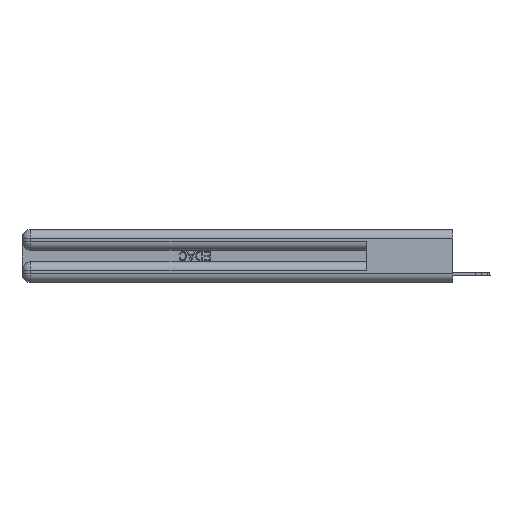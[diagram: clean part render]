
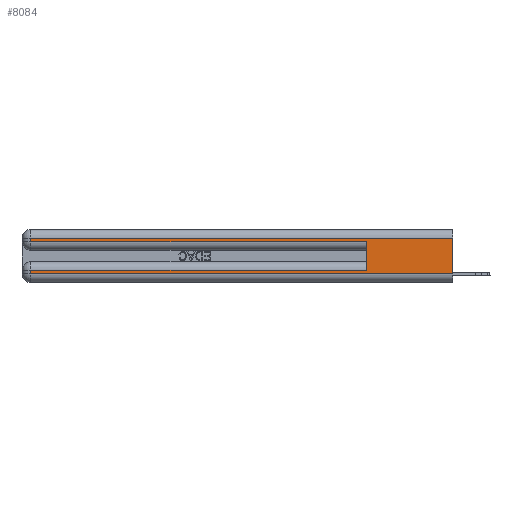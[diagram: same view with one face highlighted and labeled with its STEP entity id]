
A CAD part, left-side view. The second image highlights one B-rep face of the part: STEP entity #8084.
In plain terms, the highlighted planar face has unit normal (-1, 0, 0).
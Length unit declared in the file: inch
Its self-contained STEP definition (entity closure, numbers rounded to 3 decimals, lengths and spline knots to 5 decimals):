
#580 = CARTESIAN_POINT ( 'NONE',  ( 0., 2.94, 0.37 ) ) ;
#921 = CARTESIAN_POINT ( 'NONE',  ( 0., 0., 0.06 ) ) ;
#997 = CARTESIAN_POINT ( 'NONE',  ( 0., 0., 0.37 ) ) ;
#1278 = EDGE_CURVE ( 'NONE', #8071, #2235, #15853, .T. ) ;
#2235 = VERTEX_POINT ( 'NONE', #9827 ) ;
#2362 = CARTESIAN_POINT ( 'NONE',  ( 0., 0., 0.06 ) ) ;
#2391 = ORIENTED_EDGE ( 'NONE', *, *, #28402, .T. ) ;
#3231 = LINE ( 'NONE', #3820, #8167 ) ;
#3665 = DIRECTION ( 'NONE',  ( 0., 0., 1. ) ) ;
#3820 = CARTESIAN_POINT ( 'NONE',  ( 0., 0.6, 0.145 ) ) ;
#3840 = VECTOR ( 'NONE', #24887, 39.37008 ) ;
#4659 = ORIENTED_EDGE ( 'NONE', *, *, #1278, .T. ) ;
#4797 = ORIENTED_EDGE ( 'NONE', *, *, #5180, .T. ) ;
#5086 = VERTEX_POINT ( 'NONE', #6696 ) ;
#5180 = EDGE_CURVE ( 'NONE', #18033, #19035, #28185, .T. ) ;
#5186 = DIRECTION ( 'NONE',  ( 0., 0., -1. ) ) ;
#5324 = VECTOR ( 'NONE', #5186, 39.37008 ) ;
#5557 = CARTESIAN_POINT ( 'NONE',  ( 0., 0., 0.37 ) ) ;
#5672 = VERTEX_POINT ( 'NONE', #11124 ) ;
#5838 = CARTESIAN_POINT ( 'NONE',  ( 0., 2.94, 0.085 ) ) ;
#6696 = CARTESIAN_POINT ( 'NONE',  ( 0., 2.94, 0.06 ) ) ;
#7881 = EDGE_CURVE ( 'NONE', #8071, #9326, #16657, .T. ) ;
#7903 = CARTESIAN_POINT ( 'NONE',  ( 0., 0., 0.31 ) ) ;
#8071 = VERTEX_POINT ( 'NONE', #7903 ) ;
#8084 = ADVANCED_FACE ( 'NONE', ( #16611 ), #14813, .F. ) ;
#8167 = VECTOR ( 'NONE', #3665, 39.37008 ) ;
#9326 = VERTEX_POINT ( 'NONE', #2362 ) ;
#9507 = ORIENTED_EDGE ( 'NONE', *, *, #9837, .T. ) ;
#9827 = CARTESIAN_POINT ( 'NONE',  ( 0., 2.94, 0.31 ) ) ;
#9837 = EDGE_CURVE ( 'NONE', #5672, #10639, #11493, .T. ) ;
#9947 = EDGE_CURVE ( 'NONE', #18033, #10639, #3231, .T. ) ;
#9996 = DIRECTION ( 'NONE',  ( 0., 0., -1. ) ) ;
#10639 = VERTEX_POINT ( 'NONE', #11618 ) ;
#11124 = CARTESIAN_POINT ( 'NONE',  ( 0., 2.94, 0.285 ) ) ;
#11217 = EDGE_CURVE ( 'NONE', #5086, #9326, #11985, .T. ) ;
#11493 = LINE ( 'NONE', #27300, #27968 ) ;
#11618 = CARTESIAN_POINT ( 'NONE',  ( 0., 0.6, 0.285 ) ) ;
#11985 = LINE ( 'NONE', #921, #28981 ) ;
#12305 = DIRECTION ( 'NONE',  ( 0., 0., -1. ) ) ;
#12438 = LINE ( 'NONE', #12720, #20201 ) ;
#12720 = CARTESIAN_POINT ( 'NONE',  ( 0., 2.94, 0.37 ) ) ;
#12856 = AXIS2_PLACEMENT_3D ( 'NONE', #5557, #18840, #12305 ) ;
#13127 = ORIENTED_EDGE ( 'NONE', *, *, #23274, .T. ) ;
#13613 = CARTESIAN_POINT ( 'NONE',  ( 0., 0., 0.31 ) ) ;
#14120 = DIRECTION ( 'NONE',  ( 0., -1., 0. ) ) ;
#14813 = PLANE ( 'NONE',  #12856 ) ;
#15853 = LINE ( 'NONE', #13613, #3840 ) ;
#16119 = DIRECTION ( 'NONE',  ( 0., 1., 0. ) ) ;
#16597 = DIRECTION ( 'NONE',  ( 0., 0., -1. ) ) ;
#16611 = FACE_OUTER_BOUND ( 'NONE', #17131, .T. ) ;
#16657 = LINE ( 'NONE', #997, #23710 ) ;
#17131 = EDGE_LOOP ( 'NONE', ( #28133, #4659, #13127, #9507, #26102, #4797, #2391, #28627 ) ) ;
#18033 = VERTEX_POINT ( 'NONE', #26033 ) ;
#18586 = LINE ( 'NONE', #580, #5324 ) ;
#18673 = VECTOR ( 'NONE', #16119, 39.37008 ) ;
#18840 = DIRECTION ( 'NONE',  ( 1., 0., 0. ) ) ;
#19035 = VERTEX_POINT ( 'NONE', #5838 ) ;
#20201 = VECTOR ( 'NONE', #16597, 39.37008 ) ;
#21026 = DIRECTION ( 'NONE',  ( 0., -1., 0. ) ) ;
#23274 = EDGE_CURVE ( 'NONE', #2235, #5672, #12438, .T. ) ;
#23710 = VECTOR ( 'NONE', #9996, 39.37008 ) ;
#24887 = DIRECTION ( 'NONE',  ( 0., 1., 0. ) ) ;
#25144 = CARTESIAN_POINT ( 'NONE',  ( 0., 0., 0.085 ) ) ;
#26033 = CARTESIAN_POINT ( 'NONE',  ( 0., 0.6, 0.085 ) ) ;
#26102 = ORIENTED_EDGE ( 'NONE', *, *, #9947, .F. ) ;
#27300 = CARTESIAN_POINT ( 'NONE',  ( 0., 0., 0.285 ) ) ;
#27968 = VECTOR ( 'NONE', #14120, 39.37008 ) ;
#28133 = ORIENTED_EDGE ( 'NONE', *, *, #7881, .F. ) ;
#28185 = LINE ( 'NONE', #25144, #18673 ) ;
#28402 = EDGE_CURVE ( 'NONE', #19035, #5086, #18586, .T. ) ;
#28627 = ORIENTED_EDGE ( 'NONE', *, *, #11217, .T. ) ;
#28981 = VECTOR ( 'NONE', #21026, 39.37008 ) ;
